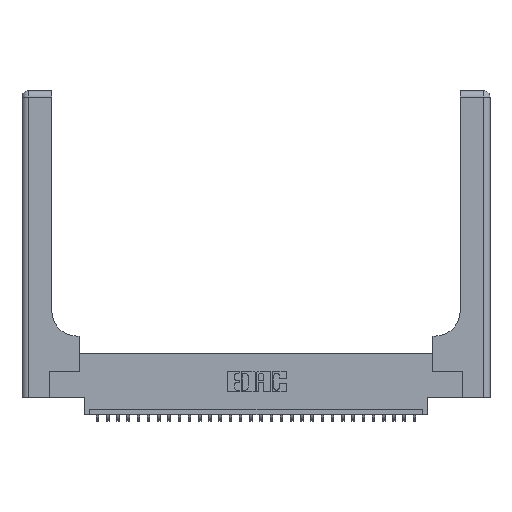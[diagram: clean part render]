
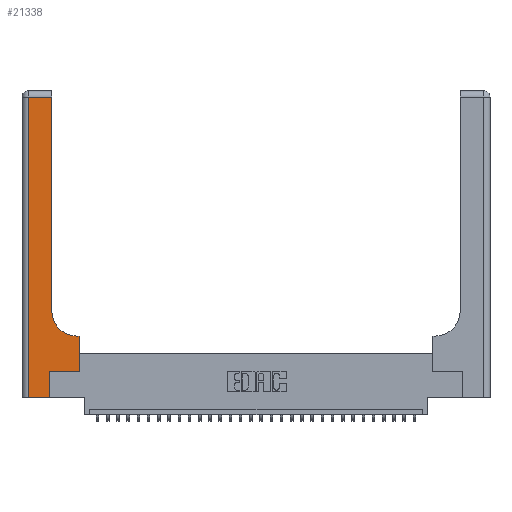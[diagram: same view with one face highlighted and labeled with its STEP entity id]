
A CAD part, top view. The second image highlights one B-rep face of the part: STEP entity #21338.
In plain terms, the highlighted planar face has unit normal (0, 0, 1).
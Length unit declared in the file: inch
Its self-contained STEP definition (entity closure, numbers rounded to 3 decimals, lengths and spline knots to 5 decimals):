
#1158 = LINE ( 'NONE', #12836, #25704 ) ;
#2262 = CARTESIAN_POINT ( 'NONE',  ( 0.269, 0., 0.37 ) ) ;
#2478 = VECTOR ( 'NONE', #6951, 39.37008 ) ;
#3061 = VERTEX_POINT ( 'NONE', #5336 ) ;
#3179 = DIRECTION ( 'NONE',  ( 1., 0., 0. ) ) ;
#3258 = VERTEX_POINT ( 'NONE', #2262 ) ;
#4109 = CARTESIAN_POINT ( 'NONE',  ( 0.5585, 0.25, 0.37 ) ) ;
#4206 = DIRECTION ( 'NONE',  ( 0., -1., 0. ) ) ;
#4386 = ORIENTED_EDGE ( 'NONE', *, *, #14147, .T. ) ;
#4432 = DIRECTION ( 'NONE',  ( 1., 0., 0. ) ) ;
#4947 = VERTEX_POINT ( 'NONE', #4109 ) ;
#5314 = PLANE ( 'NONE',  #25241 ) ;
#5336 = CARTESIAN_POINT ( 'NONE',  ( 0.5585, 0.6, 0.37 ) ) ;
#5679 = EDGE_CURVE ( 'NONE', #4947, #3061, #1158, .T. ) ;
#6223 = VERTEX_POINT ( 'NONE', #10536 ) ;
#6695 = LINE ( 'NONE', #19917, #24913 ) ;
#6951 = DIRECTION ( 'NONE',  ( 0., 1., 0. ) ) ;
#7627 = ORIENTED_EDGE ( 'NONE', *, *, #24294, .T. ) ;
#7704 = CARTESIAN_POINT ( 'NONE',  ( 0., 3., 0.37 ) ) ;
#8994 = CARTESIAN_POINT ( 'NONE',  ( 0.269, 0.25, 0.37 ) ) ;
#9421 = AXIS2_PLACEMENT_3D ( 'NONE', #17462, #29181, #3179 ) ;
#10536 = CARTESIAN_POINT ( 'NONE',  ( 0.5415, 0.6, 0.37 ) ) ;
#10752 = EDGE_LOOP ( 'NONE', ( #4386, #24743, #24360, #15196, #21708, #7627, #13120, #11962, #20018 ) ) ;
#10764 = VECTOR ( 'NONE', #29863, 39.37008 ) ;
#11962 = ORIENTED_EDGE ( 'NONE', *, *, #19132, .T. ) ;
#12836 = CARTESIAN_POINT ( 'NONE',  ( 0.5585, 0.25, 0.37 ) ) ;
#13120 = ORIENTED_EDGE ( 'NONE', *, *, #5679, .T. ) ;
#13145 = DIRECTION ( 'NONE',  ( 0., 1., 0. ) ) ;
#13268 = CARTESIAN_POINT ( 'NONE',  ( 0.06, 0., 0.37 ) ) ;
#13731 = VERTEX_POINT ( 'NONE', #21292 ) ;
#14015 = CARTESIAN_POINT ( 'NONE',  ( 0.2915, 3., 0.37 ) ) ;
#14146 = DIRECTION ( 'NONE',  ( -1., 0., 0. ) ) ;
#14147 = EDGE_CURVE ( 'NONE', #13731, #16519, #21066, .T. ) ;
#15080 = DIRECTION ( 'NONE',  ( -1., 0., 0. ) ) ;
#15196 = ORIENTED_EDGE ( 'NONE', *, *, #25476, .T. ) ;
#15471 = CARTESIAN_POINT ( 'NONE',  ( 0.269, 0., 0.37 ) ) ;
#15491 = VERTEX_POINT ( 'NONE', #13268 ) ;
#15798 = VECTOR ( 'NONE', #4206, 39.37008 ) ;
#16181 = CARTESIAN_POINT ( 'NONE',  ( 0.06, 3., 0.37 ) ) ;
#16432 = VECTOR ( 'NONE', #4432, 39.37008 ) ;
#16519 = VERTEX_POINT ( 'NONE', #18122 ) ;
#16589 = VECTOR ( 'NONE', #21735, 39.37008 ) ;
#17462 = CARTESIAN_POINT ( 'NONE',  ( 0.5415, 0.85, 0.37 ) ) ;
#17490 = EDGE_CURVE ( 'NONE', #16519, #19002, #30198, .T. ) ;
#17737 = CARTESIAN_POINT ( 'NONE',  ( 0.2915, 0.6, 0.37 ) ) ;
#18069 = LINE ( 'NONE', #16181, #15798 ) ;
#18122 = CARTESIAN_POINT ( 'NONE',  ( 0.2915, 2.94, 0.37 ) ) ;
#18381 = CARTESIAN_POINT ( 'NONE',  ( 0.269, 0.25, 0.37 ) ) ;
#18500 = LINE ( 'NONE', #8994, #16432 ) ;
#19002 = VERTEX_POINT ( 'NONE', #28702 ) ;
#19132 = EDGE_CURVE ( 'NONE', #3061, #6223, #24529, .T. ) ;
#19917 = CARTESIAN_POINT ( 'NONE',  ( 0., 0., 0.37 ) ) ;
#20018 = ORIENTED_EDGE ( 'NONE', *, *, #29101, .T. ) ;
#21066 = LINE ( 'NONE', #14015, #2478 ) ;
#21292 = CARTESIAN_POINT ( 'NONE',  ( 0.2915, 0.85, 0.37 ) ) ;
#21338 = ADVANCED_FACE ( 'NONE', ( #28144 ), #5314, .F. ) ;
#21708 = ORIENTED_EDGE ( 'NONE', *, *, #22011, .T. ) ;
#21735 = DIRECTION ( 'NONE',  ( 0., 1., 0. ) ) ;
#22011 = EDGE_CURVE ( 'NONE', #3258, #28841, #22902, .T. ) ;
#22395 = VECTOR ( 'NONE', #14146, 39.37008 ) ;
#22902 = LINE ( 'NONE', #15471, #16589 ) ;
#24294 = EDGE_CURVE ( 'NONE', #28841, #4947, #18500, .T. ) ;
#24360 = ORIENTED_EDGE ( 'NONE', *, *, #28931, .T. ) ;
#24529 = LINE ( 'NONE', #17737, #10764 ) ;
#24743 = ORIENTED_EDGE ( 'NONE', *, *, #17490, .T. ) ;
#24913 = VECTOR ( 'NONE', #29557, 39.37008 ) ;
#25241 = AXIS2_PLACEMENT_3D ( 'NONE', #7704, #26941, #15080 ) ;
#25476 = EDGE_CURVE ( 'NONE', #15491, #3258, #6695, .T. ) ;
#25704 = VECTOR ( 'NONE', #13145, 39.37008 ) ;
#26941 = DIRECTION ( 'NONE',  ( 0., 0., -1. ) ) ;
#28144 = FACE_OUTER_BOUND ( 'NONE', #10752, .T. ) ;
#28702 = CARTESIAN_POINT ( 'NONE',  ( 0.06, 2.94, 0.37 ) ) ;
#28841 = VERTEX_POINT ( 'NONE', #18381 ) ;
#28931 = EDGE_CURVE ( 'NONE', #19002, #15491, #18069, .T. ) ;
#29101 = EDGE_CURVE ( 'NONE', #6223, #13731, #30311, .T. ) ;
#29181 = DIRECTION ( 'NONE',  ( 0., 0., -1. ) ) ;
#29557 = DIRECTION ( 'NONE',  ( 1., 0., 0. ) ) ;
#29863 = DIRECTION ( 'NONE',  ( -1., 0., 0. ) ) ;
#30198 = LINE ( 'NONE', #30589, #22395 ) ;
#30311 = CIRCLE ( 'NONE', #9421, 0.25 ) ;
#30589 = CARTESIAN_POINT ( 'NONE',  ( 0., 2.94, 0.37 ) ) ;
